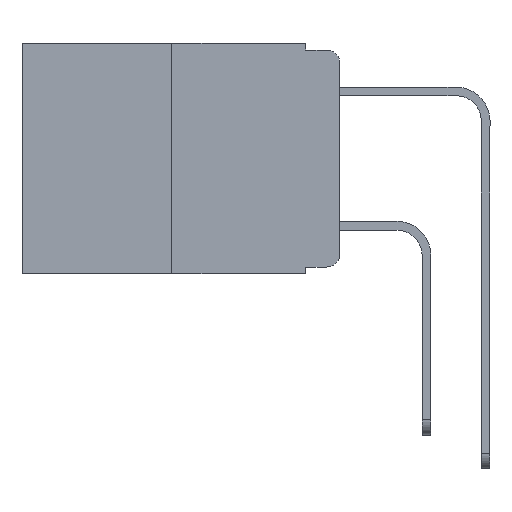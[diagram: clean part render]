
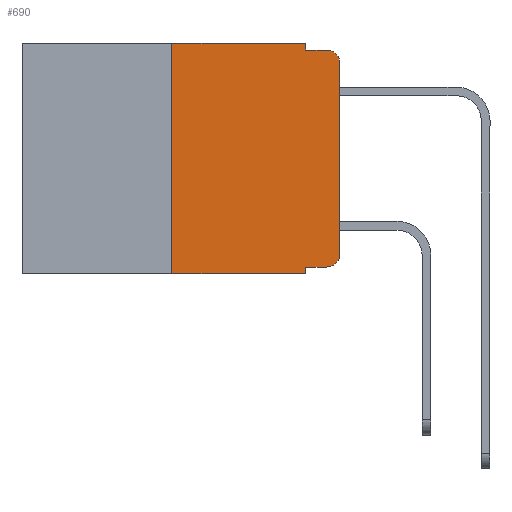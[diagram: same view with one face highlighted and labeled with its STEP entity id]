
A CAD part, left-side view. The second image highlights one B-rep face of the part: STEP entity #690.
In plain terms, the highlighted planar face has unit normal (-1, 0, 0).
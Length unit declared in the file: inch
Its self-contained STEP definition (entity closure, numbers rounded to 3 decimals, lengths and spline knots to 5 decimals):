
#479 = VECTOR ( 'NONE', #12119, 39.37008 ) ;
#487 = VERTEX_POINT ( 'NONE', #4157 ) ;
#661 = CARTESIAN_POINT ( 'NONE',  ( 0., 0.051, -0.01 ) ) ;
#690 = ADVANCED_FACE ( 'NONE', ( #4577 ), #1062, .F. ) ;
#718 = EDGE_CURVE ( 'NONE', #13507, #7178, #1637, .T. ) ;
#940 = CARTESIAN_POINT ( 'NONE',  ( 0., 0.25, 0. ) ) ;
#949 = CARTESIAN_POINT ( 'NONE',  ( 0., 0.25, -0.343 ) ) ;
#1007 = CARTESIAN_POINT ( 'NONE',  ( 0., 0.02, -0.03 ) ) ;
#1062 = PLANE ( 'NONE',  #2960 ) ;
#1393 = VERTEX_POINT ( 'NONE', #5962 ) ;
#1637 = LINE ( 'NONE', #940, #12653 ) ;
#2089 = VECTOR ( 'NONE', #12221, 39.37008 ) ;
#2138 = DIRECTION ( 'NONE',  ( 0., 0., -1. ) ) ;
#2244 = AXIS2_PLACEMENT_3D ( 'NONE', #1007, #8785, #2138 ) ;
#2876 = VECTOR ( 'NONE', #4443, 39.37008 ) ;
#2940 = CARTESIAN_POINT ( 'NONE',  ( 0., 0.051, 0. ) ) ;
#2960 = AXIS2_PLACEMENT_3D ( 'NONE', #8243, #4767, #8648 ) ;
#3013 = EDGE_CURVE ( 'NONE', #10154, #8430, #6050, .T. ) ;
#3075 = CIRCLE ( 'NONE', #2244, 0.02 ) ;
#3085 = EDGE_CURVE ( 'NONE', #7952, #1393, #5024, .T. ) ;
#3280 = LINE ( 'NONE', #8602, #9141 ) ;
#3336 = CARTESIAN_POINT ( 'NONE',  ( 0., 0.051, -0.333 ) ) ;
#3348 = CARTESIAN_POINT ( 'NONE',  ( 0., 0.473, 0. ) ) ;
#3607 = CARTESIAN_POINT ( 'NONE',  ( 0., 0.02, -0.333 ) ) ;
#3906 = CARTESIAN_POINT ( 'NONE',  ( 0., 0.051, 0. ) ) ;
#4023 = ORIENTED_EDGE ( 'NONE', *, *, #6348, .T. ) ;
#4157 = CARTESIAN_POINT ( 'NONE',  ( 0., 0.051, -0.343 ) ) ;
#4207 = ORIENTED_EDGE ( 'NONE', *, *, #13856, .T. ) ;
#4427 = ORIENTED_EDGE ( 'NONE', *, *, #5934, .F. ) ;
#4443 = DIRECTION ( 'NONE',  ( 0., -1., 0. ) ) ;
#4577 = FACE_OUTER_BOUND ( 'NONE', #11812, .T. ) ;
#4619 = EDGE_CURVE ( 'NONE', #4652, #6089, #3280, .T. ) ;
#4652 = VERTEX_POINT ( 'NONE', #8649 ) ;
#4767 = DIRECTION ( 'NONE',  ( 1., 0., 0. ) ) ;
#4925 = CARTESIAN_POINT ( 'NONE',  ( 0., 0.473, -0.343 ) ) ;
#5024 = LINE ( 'NONE', #5622, #2089 ) ;
#5155 = DIRECTION ( 'NONE',  ( 0., 0., -1. ) ) ;
#5199 = DIRECTION ( 'NONE',  ( -1., 0., 0. ) ) ;
#5268 = EDGE_CURVE ( 'NONE', #6089, #13718, #3075, .T. ) ;
#5347 = ORIENTED_EDGE ( 'NONE', *, *, #718, .F. ) ;
#5580 = AXIS2_PLACEMENT_3D ( 'NONE', #11791, #5199, #12897 ) ;
#5622 = CARTESIAN_POINT ( 'NONE',  ( 0., 0.051, 0. ) ) ;
#5675 = CIRCLE ( 'NONE', #5580, 0.02 ) ;
#5934 = EDGE_CURVE ( 'NONE', #7178, #7952, #11651, .T. ) ;
#5957 = ORIENTED_EDGE ( 'NONE', *, *, #3013, .T. ) ;
#5962 = CARTESIAN_POINT ( 'NONE',  ( 0., 0.051, -0.01 ) ) ;
#6050 = LINE ( 'NONE', #3336, #479 ) ;
#6089 = VERTEX_POINT ( 'NONE', #13434 ) ;
#6327 = EDGE_CURVE ( 'NONE', #10154, #487, #13723, .T. ) ;
#6348 = EDGE_CURVE ( 'NONE', #8430, #4652, #5675, .T. ) ;
#6701 = ORIENTED_EDGE ( 'NONE', *, *, #10824, .F. ) ;
#7178 = VERTEX_POINT ( 'NONE', #8999 ) ;
#7236 = CARTESIAN_POINT ( 'NONE',  ( 0., 0.051, -0.333 ) ) ;
#7318 = DIRECTION ( 'NONE',  ( 0., -1., 0. ) ) ;
#7952 = VERTEX_POINT ( 'NONE', #3906 ) ;
#8051 = ORIENTED_EDGE ( 'NONE', *, *, #5268, .T. ) ;
#8079 = DIRECTION ( 'NONE',  ( 0., 0., 1. ) ) ;
#8198 = ORIENTED_EDGE ( 'NONE', *, *, #6327, .F. ) ;
#8243 = CARTESIAN_POINT ( 'NONE',  ( 0., 0.473, 0. ) ) ;
#8430 = VERTEX_POINT ( 'NONE', #3607 ) ;
#8602 = CARTESIAN_POINT ( 'NONE',  ( 0., 0., 0. ) ) ;
#8648 = DIRECTION ( 'NONE',  ( 0., 0., -1. ) ) ;
#8649 = CARTESIAN_POINT ( 'NONE',  ( 0., 0., -0.313 ) ) ;
#8700 = LINE ( 'NONE', #4925, #13766 ) ;
#8785 = DIRECTION ( 'NONE',  ( -1., 0., 0. ) ) ;
#8999 = CARTESIAN_POINT ( 'NONE',  ( 0., 0.25, 0. ) ) ;
#9141 = VECTOR ( 'NONE', #10740, 39.37008 ) ;
#9494 = ORIENTED_EDGE ( 'NONE', *, *, #4619, .T. ) ;
#9556 = VECTOR ( 'NONE', #7318, 39.37008 ) ;
#9911 = LINE ( 'NONE', #661, #9556 ) ;
#10154 = VERTEX_POINT ( 'NONE', #7236 ) ;
#10740 = DIRECTION ( 'NONE',  ( 0., 0., 1. ) ) ;
#10824 = EDGE_CURVE ( 'NONE', #1393, #13718, #9911, .T. ) ;
#11191 = VECTOR ( 'NONE', #5155, 39.37008 ) ;
#11651 = LINE ( 'NONE', #3348, #2876 ) ;
#11791 = CARTESIAN_POINT ( 'NONE',  ( 0., 0.02, -0.313 ) ) ;
#11812 = EDGE_LOOP ( 'NONE', ( #9494, #8051, #6701, #12577, #4427, #5347, #4207, #8198, #5957, #4023 ) ) ;
#12119 = DIRECTION ( 'NONE',  ( 0., -1., 0. ) ) ;
#12221 = DIRECTION ( 'NONE',  ( 0., 0., -1. ) ) ;
#12377 = CARTESIAN_POINT ( 'NONE',  ( 0., 0.02, -0.01 ) ) ;
#12577 = ORIENTED_EDGE ( 'NONE', *, *, #3085, .F. ) ;
#12653 = VECTOR ( 'NONE', #8079, 39.37008 ) ;
#12897 = DIRECTION ( 'NONE',  ( 0., 0., -1. ) ) ;
#13434 = CARTESIAN_POINT ( 'NONE',  ( 0., 0., -0.03 ) ) ;
#13507 = VERTEX_POINT ( 'NONE', #949 ) ;
#13683 = DIRECTION ( 'NONE',  ( 0., -1., 0. ) ) ;
#13718 = VERTEX_POINT ( 'NONE', #12377 ) ;
#13723 = LINE ( 'NONE', #2940, #11191 ) ;
#13766 = VECTOR ( 'NONE', #13683, 39.37008 ) ;
#13856 = EDGE_CURVE ( 'NONE', #13507, #487, #8700, .T. ) ;
